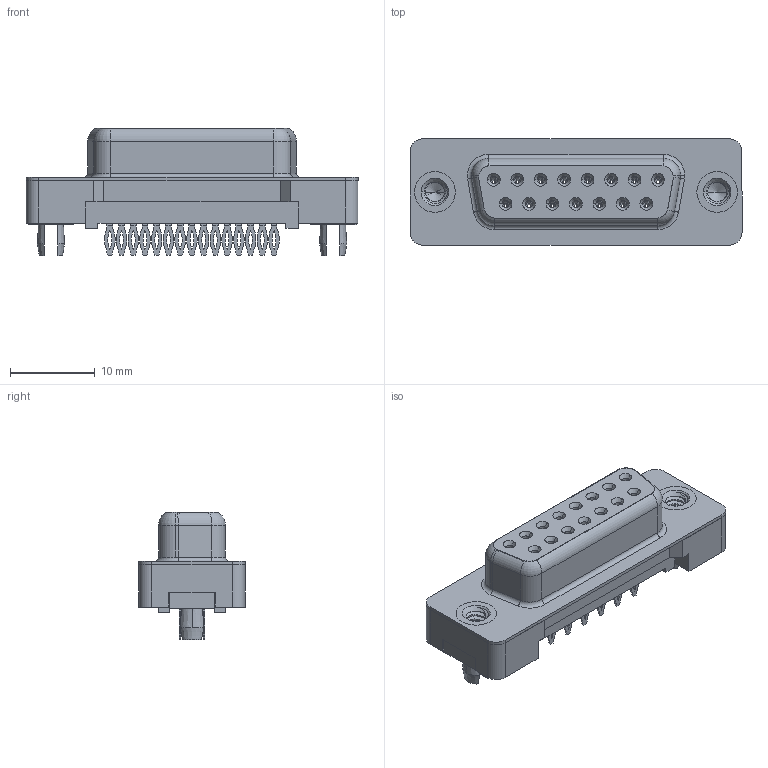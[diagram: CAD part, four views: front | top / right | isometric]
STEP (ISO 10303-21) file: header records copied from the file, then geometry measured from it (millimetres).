
FILE_DESCRIPTION (( 'STEP AP203' ), '1' );
FILE_NAME ('628-015-226-016.STEP', '2020-07-15T23:11:47', ( '' ), ( '' ), 'SwSTEP 2.0', 'SolidWorks 2020', '' );
FILE_SCHEMA (( 'CONFIG_CONTROL_DESIGN' ));
Length unit declared in the file: millimetre
Products named in the file (6): 628 PB Contact Row 1_26; 628 PB Shell_15 Contacts; 628 PB 4-40 Threaded Rivet with Boardlock; 628 PB Contact Row 2_26; 628 Plastic Body Housing_15 Contacts; 628-015-226-016
Assembly tree (19 placements, depth 2):
  628-015-226-016
    628 Plastic Body Housing_15 Contacts
    628 PB Shell_15 Contacts
    628 PB Contact Row 1_26  x8
    628 PB Contact Row 2_26  x7
    628 PB 4-40 Threaded Rivet with Boardlock  x2
Bounding box: 39.2 x 12.55 x 15.05 mm (x, y, z)
Volume: 2482.1 mm3; surface area: 5979.3 mm2
Topology: 19 solids, 19 shells, 1611 faces, 3941 edges, 2396 vertices
Faces by surface type: plane 664, cylinder 398, bspline 336, torus 116, cone 97
Entity records: 18618 total; most frequent: CARTESIAN_POINT 5657, ORIENTED_EDGE 2524, DIRECTION 2395, EDGE_CURVE 1262, AXIS2_PLACEMENT_3D 825, VERTEX_POINT 787, LINE 745, VECTOR 745
